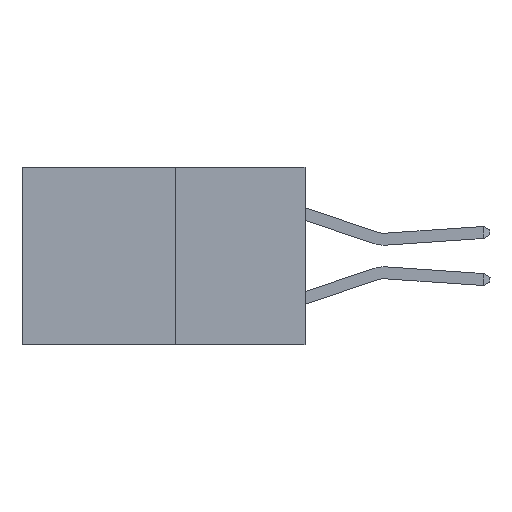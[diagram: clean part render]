
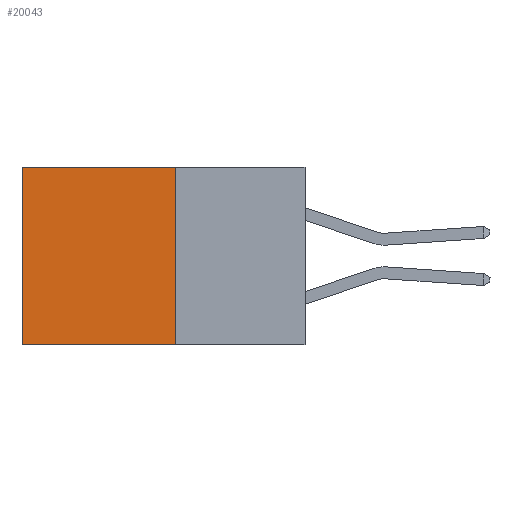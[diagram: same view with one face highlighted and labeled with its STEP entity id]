
A CAD part, left-side view. The second image highlights one B-rep face of the part: STEP entity #20043.
In plain terms, the highlighted planar face has unit normal (-1, 0, 0).
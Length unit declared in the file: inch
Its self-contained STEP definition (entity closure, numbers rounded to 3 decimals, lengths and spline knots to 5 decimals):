
#447 = VECTOR ( 'NONE', #3231, 39.37008 ) ;
#1509 = CARTESIAN_POINT ( 'NONE',  ( 0.277, 0.27, -0.37 ) ) ;
#2905 = VERTEX_POINT ( 'NONE', #8729 ) ;
#2966 = CARTESIAN_POINT ( 'NONE',  ( 0.277, 0.27, -0.37 ) ) ;
#3231 = DIRECTION ( 'NONE',  ( 0., 1., 0. ) ) ;
#3884 = ORIENTED_EDGE ( 'NONE', *, *, #10424, .F. ) ;
#5450 = ORIENTED_EDGE ( 'NONE', *, *, #8181, .T. ) ;
#5634 = CARTESIAN_POINT ( 'NONE',  ( 0.277, 0.27, -0.37 ) ) ;
#5967 = LINE ( 'NONE', #2966, #30816 ) ;
#7023 = AXIS2_PLACEMENT_3D ( 'NONE', #10076, #29278, #14997 ) ;
#8094 = CARTESIAN_POINT ( 'NONE',  ( 0.277, 0.59, 0. ) ) ;
#8181 = EDGE_CURVE ( 'NONE', #14074, #15049, #13488, .T. ) ;
#8729 = CARTESIAN_POINT ( 'NONE',  ( 0.277, 0.59, -0.37 ) ) ;
#10076 = CARTESIAN_POINT ( 'NONE',  ( 0.277, 0.27, -0.37 ) ) ;
#10424 = EDGE_CURVE ( 'NONE', #21416, #2905, #28735, .T. ) ;
#11509 = DIRECTION ( 'NONE',  ( 0., 0., -1. ) ) ;
#12520 = PLANE ( 'NONE',  #7023 ) ;
#13488 = LINE ( 'NONE', #20280, #447 ) ;
#14074 = VERTEX_POINT ( 'NONE', #22901 ) ;
#14997 = DIRECTION ( 'NONE',  ( 0., 0., -1. ) ) ;
#15049 = VERTEX_POINT ( 'NONE', #8094 ) ;
#15857 = ORIENTED_EDGE ( 'NONE', *, *, #22762, .F. ) ;
#15973 = VECTOR ( 'NONE', #11509, 39.37008 ) ;
#19457 = FACE_OUTER_BOUND ( 'NONE', #29668, .T. ) ;
#20011 = DIRECTION ( 'NONE',  ( 0., 0., -1. ) ) ;
#20043 = ADVANCED_FACE ( 'NONE', ( #19457 ), #12520, .F. ) ;
#20280 = CARTESIAN_POINT ( 'NONE',  ( 0.277, 0.27, 0. ) ) ;
#20943 = VECTOR ( 'NONE', #23280, 39.37008 ) ;
#21416 = VERTEX_POINT ( 'NONE', #5634 ) ;
#22762 = EDGE_CURVE ( 'NONE', #14074, #21416, #5967, .T. ) ;
#22901 = CARTESIAN_POINT ( 'NONE',  ( 0.277, 0.27, 0. ) ) ;
#23280 = DIRECTION ( 'NONE',  ( 0., 1., 0. ) ) ;
#27358 = ORIENTED_EDGE ( 'NONE', *, *, #27754, .T. ) ;
#27754 = EDGE_CURVE ( 'NONE', #15049, #2905, #29387, .T. ) ;
#28265 = CARTESIAN_POINT ( 'NONE',  ( 0.277, 0.59, -0.37 ) ) ;
#28735 = LINE ( 'NONE', #1509, #20943 ) ;
#29278 = DIRECTION ( 'NONE',  ( 1., 0., 0. ) ) ;
#29387 = LINE ( 'NONE', #28265, #15973 ) ;
#29668 = EDGE_LOOP ( 'NONE', ( #27358, #3884, #15857, #5450 ) ) ;
#30816 = VECTOR ( 'NONE', #20011, 39.37008 ) ;
